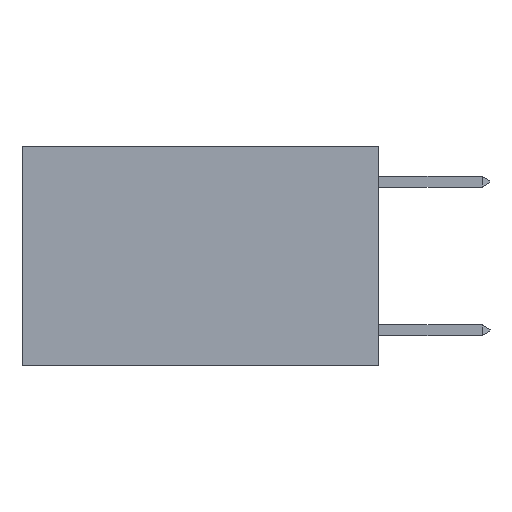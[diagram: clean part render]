
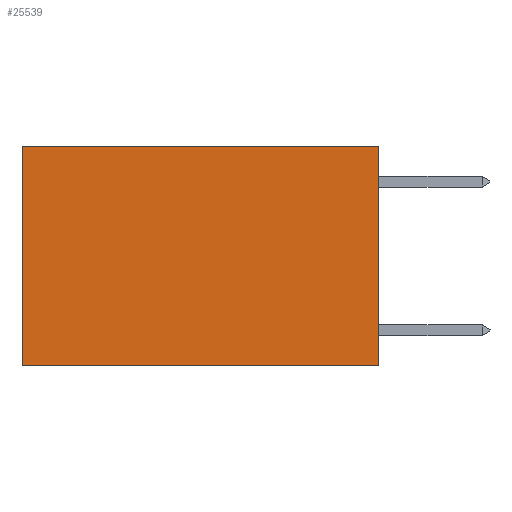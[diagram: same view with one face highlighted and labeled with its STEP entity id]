
A CAD part, left-side view. The second image highlights one B-rep face of the part: STEP entity #25539.
In plain terms, the highlighted planar face has unit normal (-1, 0, 0).
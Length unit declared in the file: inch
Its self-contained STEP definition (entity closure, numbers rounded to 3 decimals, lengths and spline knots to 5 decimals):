
#201 = DIRECTION ( 'NONE',  ( 0., 0., -1. ) ) ;
#626 = DIRECTION ( 'NONE',  ( 0., 1., 0. ) ) ;
#776 = LINE ( 'NONE', #22682, #10320 ) ;
#1588 = VECTOR ( 'NONE', #20652, 39.37008 ) ;
#1720 = CARTESIAN_POINT ( 'NONE',  ( 0.2625, 0., 0. ) ) ;
#2535 = PLANE ( 'NONE',  #9262 ) ;
#4015 = CARTESIAN_POINT ( 'NONE',  ( 0.2625, 0.6, -0.37 ) ) ;
#6360 = CARTESIAN_POINT ( 'NONE',  ( 0.2625, 0.6, 0. ) ) ;
#7300 = EDGE_CURVE ( 'NONE', #7984, #22963, #25737, .T. ) ;
#7984 = VERTEX_POINT ( 'NONE', #6360 ) ;
#8817 = VECTOR ( 'NONE', #21122, 39.37008 ) ;
#8865 = DIRECTION ( 'NONE',  ( 0., 0., -1. ) ) ;
#9230 = DIRECTION ( 'NONE',  ( 1., 0., 0. ) ) ;
#9262 = AXIS2_PLACEMENT_3D ( 'NONE', #11708, #9230, #201 ) ;
#9440 = CARTESIAN_POINT ( 'NONE',  ( 0.2625, 0., -0.37 ) ) ;
#10320 = VECTOR ( 'NONE', #8865, 39.37008 ) ;
#11708 = CARTESIAN_POINT ( 'NONE',  ( 0.2625, 0., 0. ) ) ;
#11901 = CARTESIAN_POINT ( 'NONE',  ( 0.2625, 0.6, 0. ) ) ;
#12236 = ORIENTED_EDGE ( 'NONE', *, *, #12993, .F. ) ;
#12637 = LINE ( 'NONE', #1720, #18108 ) ;
#12993 = EDGE_CURVE ( 'NONE', #13349, #22963, #18435, .T. ) ;
#13327 = VERTEX_POINT ( 'NONE', #25794 ) ;
#13349 = VERTEX_POINT ( 'NONE', #9440 ) ;
#14260 = EDGE_CURVE ( 'NONE', #13327, #13349, #776, .T. ) ;
#14974 = EDGE_LOOP ( 'NONE', ( #15039, #12236, #22623, #30029 ) ) ;
#15039 = ORIENTED_EDGE ( 'NONE', *, *, #7300, .T. ) ;
#18108 = VECTOR ( 'NONE', #626, 39.37008 ) ;
#18435 = LINE ( 'NONE', #22740, #1588 ) ;
#20194 = FACE_OUTER_BOUND ( 'NONE', #14974, .T. ) ;
#20652 = DIRECTION ( 'NONE',  ( 0., 1., 0. ) ) ;
#21122 = DIRECTION ( 'NONE',  ( 0., 0., -1. ) ) ;
#22623 = ORIENTED_EDGE ( 'NONE', *, *, #14260, .F. ) ;
#22682 = CARTESIAN_POINT ( 'NONE',  ( 0.2625, 0., 0. ) ) ;
#22740 = CARTESIAN_POINT ( 'NONE',  ( 0.2625, 0., -0.37 ) ) ;
#22963 = VERTEX_POINT ( 'NONE', #4015 ) ;
#25539 = ADVANCED_FACE ( 'NONE', ( #20194 ), #2535, .F. ) ;
#25737 = LINE ( 'NONE', #11901, #8817 ) ;
#25794 = CARTESIAN_POINT ( 'NONE',  ( 0.2625, 0., 0. ) ) ;
#30029 = ORIENTED_EDGE ( 'NONE', *, *, #30285, .T. ) ;
#30285 = EDGE_CURVE ( 'NONE', #13327, #7984, #12637, .T. ) ;
